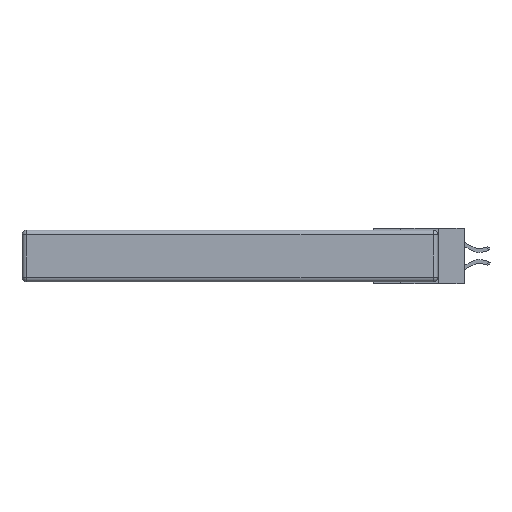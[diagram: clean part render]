
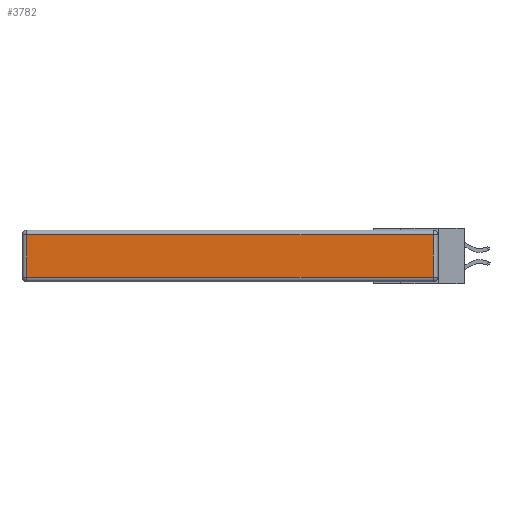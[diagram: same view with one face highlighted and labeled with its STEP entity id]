
A CAD part, left-side view. The second image highlights one B-rep face of the part: STEP entity #3782.
In plain terms, the highlighted planar face has unit normal (-1, 0, 0).
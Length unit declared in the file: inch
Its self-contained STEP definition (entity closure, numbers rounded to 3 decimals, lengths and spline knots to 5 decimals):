
#160 = CARTESIAN_POINT ( 'NONE',  ( 0., 2.72, -0.343 ) ) ;
#487 = CARTESIAN_POINT ( 'NONE',  ( 0., 2.72, -0.313 ) ) ;
#902 = VERTEX_POINT ( 'NONE', #487 ) ;
#1308 = EDGE_CURVE ( 'NONE', #6817, #902, #7405, .T. ) ;
#1793 = DIRECTION ( 'NONE',  ( -1., 0., 0. ) ) ;
#2335 = VECTOR ( 'NONE', #10799, 39.37008 ) ;
#2488 = CARTESIAN_POINT ( 'NONE',  ( 0., 0.03, -0.343 ) ) ;
#2747 = CARTESIAN_POINT ( 'NONE',  ( 0., 2.75, -0.03 ) ) ;
#2973 = ORIENTED_EDGE ( 'NONE', *, *, #9348, .T. ) ;
#3281 = VERTEX_POINT ( 'NONE', #3726 ) ;
#3468 = LINE ( 'NONE', #3927, #9925 ) ;
#3706 = VECTOR ( 'NONE', #7929, 39.37008 ) ;
#3726 = CARTESIAN_POINT ( 'NONE',  ( 0., 0.03, -0.313 ) ) ;
#3782 = ADVANCED_FACE ( 'NONE', ( #6549 ), #6125, .T. ) ;
#3791 = DIRECTION ( 'NONE',  ( 0., -1., 0. ) ) ;
#3927 = CARTESIAN_POINT ( 'NONE',  ( 0., 0., -0.313 ) ) ;
#4691 = CARTESIAN_POINT ( 'NONE',  ( 0., 2.72, -0.03 ) ) ;
#6097 = ORIENTED_EDGE ( 'NONE', *, *, #7970, .T. ) ;
#6125 = PLANE ( 'NONE',  #6446 ) ;
#6446 = AXIS2_PLACEMENT_3D ( 'NONE', #13644, #1793, #13498 ) ;
#6498 = LINE ( 'NONE', #2747, #3706 ) ;
#6549 = FACE_OUTER_BOUND ( 'NONE', #6985, .T. ) ;
#6660 = EDGE_CURVE ( 'NONE', #3281, #11409, #9284, .T. ) ;
#6817 = VERTEX_POINT ( 'NONE', #4691 ) ;
#6985 = EDGE_LOOP ( 'NONE', ( #6097, #12998, #2973, #9400 ) ) ;
#7405 = LINE ( 'NONE', #160, #13500 ) ;
#7929 = DIRECTION ( 'NONE',  ( 0., 1., 0. ) ) ;
#7970 = EDGE_CURVE ( 'NONE', #902, #3281, #3468, .T. ) ;
#9284 = LINE ( 'NONE', #2488, #2335 ) ;
#9348 = EDGE_CURVE ( 'NONE', #11409, #6817, #6498, .T. ) ;
#9400 = ORIENTED_EDGE ( 'NONE', *, *, #1308, .T. ) ;
#9925 = VECTOR ( 'NONE', #3791, 39.37008 ) ;
#10799 = DIRECTION ( 'NONE',  ( 0., 0., 1. ) ) ;
#11382 = CARTESIAN_POINT ( 'NONE',  ( 0., 0.03, -0.03 ) ) ;
#11409 = VERTEX_POINT ( 'NONE', #11382 ) ;
#11780 = DIRECTION ( 'NONE',  ( 0., 0., -1. ) ) ;
#12998 = ORIENTED_EDGE ( 'NONE', *, *, #6660, .T. ) ;
#13498 = DIRECTION ( 'NONE',  ( 0., 0., 1. ) ) ;
#13500 = VECTOR ( 'NONE', #11780, 39.37008 ) ;
#13644 = CARTESIAN_POINT ( 'NONE',  ( 0., 0., -0.343 ) ) ;
